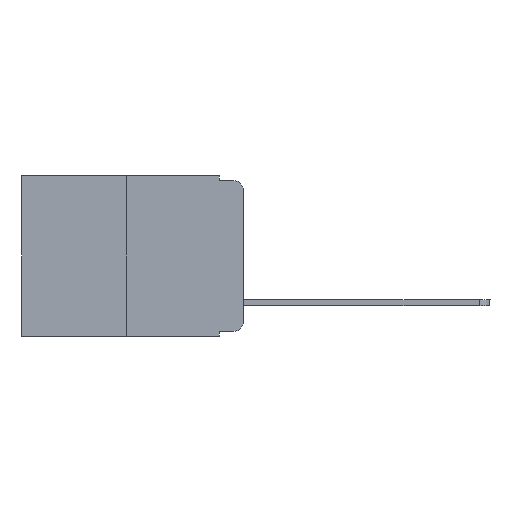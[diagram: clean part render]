
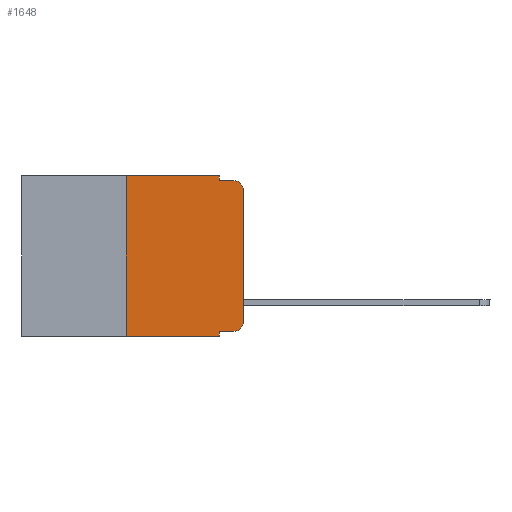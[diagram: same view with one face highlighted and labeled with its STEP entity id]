
A CAD part, left-side view. The second image highlights one B-rep face of the part: STEP entity #1648.
In plain terms, the highlighted planar face has unit normal (-1, 0, 0).
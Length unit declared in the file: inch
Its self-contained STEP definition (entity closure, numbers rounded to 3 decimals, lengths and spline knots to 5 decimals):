
#95 = LINE ( 'NONE', #11954, #1100 ) ;
#121 = VERTEX_POINT ( 'NONE', #2154 ) ;
#850 = ORIENTED_EDGE ( 'NONE', *, *, #11489, .T. ) ;
#967 = LINE ( 'NONE', #10029, #12009 ) ;
#1044 = CARTESIAN_POINT ( 'NONE',  ( 0., 0.02, -0.313 ) ) ;
#1087 = EDGE_CURVE ( 'NONE', #8851, #10928, #6207, .T. ) ;
#1100 = VECTOR ( 'NONE', #3570, 39.37008 ) ;
#1183 = VERTEX_POINT ( 'NONE', #7069 ) ;
#1648 = ADVANCED_FACE ( 'NONE', ( #4651 ), #10179, .F. ) ;
#1920 = DIRECTION ( 'NONE',  ( 0., 0., -1. ) ) ;
#1926 = AXIS2_PLACEMENT_3D ( 'NONE', #1044, #13629, #8366 ) ;
#1992 = EDGE_CURVE ( 'NONE', #7765, #7007, #9075, .T. ) ;
#2034 = EDGE_CURVE ( 'NONE', #4441, #1183, #13520, .T. ) ;
#2062 = CARTESIAN_POINT ( 'NONE',  ( 0., 0.02, -0.03 ) ) ;
#2102 = LINE ( 'NONE', #10497, #10202 ) ;
#2111 = CARTESIAN_POINT ( 'NONE',  ( 0., 0.25, 0. ) ) ;
#2154 = CARTESIAN_POINT ( 'NONE',  ( 0., 0.051, -0.333 ) ) ;
#3027 = CARTESIAN_POINT ( 'NONE',  ( 0., 0., -0.313 ) ) ;
#3145 = CARTESIAN_POINT ( 'NONE',  ( 0., 0.02, -0.333 ) ) ;
#3453 = CARTESIAN_POINT ( 'NONE',  ( 0., 0., -0.03 ) ) ;
#3570 = DIRECTION ( 'NONE',  ( 0., -1., 0. ) ) ;
#3577 = VECTOR ( 'NONE', #4311, 39.37008 ) ;
#3691 = EDGE_CURVE ( 'NONE', #121, #7007, #967, .T. ) ;
#3725 = CARTESIAN_POINT ( 'NONE',  ( 0., 0.25, -0.343 ) ) ;
#3776 = ORIENTED_EDGE ( 'NONE', *, *, #1087, .T. ) ;
#4140 = CARTESIAN_POINT ( 'NONE',  ( 0., 0.051, 0. ) ) ;
#4193 = ORIENTED_EDGE ( 'NONE', *, *, #8775, .T. ) ;
#4295 = VERTEX_POINT ( 'NONE', #4140 ) ;
#4311 = DIRECTION ( 'NONE',  ( 0., -1., 0. ) ) ;
#4322 = CARTESIAN_POINT ( 'NONE',  ( 0., 0.051, -0.01 ) ) ;
#4402 = DIRECTION ( 'NONE',  ( 0., -1., 0. ) ) ;
#4441 = VERTEX_POINT ( 'NONE', #4322 ) ;
#4563 = EDGE_CURVE ( 'NONE', #10100, #4295, #95, .T. ) ;
#4588 = ORIENTED_EDGE ( 'NONE', *, *, #13112, .T. ) ;
#4651 = FACE_OUTER_BOUND ( 'NONE', #6833, .T. ) ;
#4959 = DIRECTION ( 'NONE',  ( 0., 0., 1. ) ) ;
#5990 = CARTESIAN_POINT ( 'NONE',  ( 0., 0.051, 0. ) ) ;
#6037 = ORIENTED_EDGE ( 'NONE', *, *, #4563, .F. ) ;
#6207 = LINE ( 'NONE', #7023, #11497 ) ;
#6371 = AXIS2_PLACEMENT_3D ( 'NONE', #2062, #12422, #1920 ) ;
#6585 = ORIENTED_EDGE ( 'NONE', *, *, #3691, .F. ) ;
#6833 = EDGE_LOOP ( 'NONE', ( #3776, #4193, #12288, #9859, #6037, #12783, #11255, #6585, #850, #4588 ) ) ;
#7007 = VERTEX_POINT ( 'NONE', #10623 ) ;
#7023 = CARTESIAN_POINT ( 'NONE',  ( 0., 0., 0. ) ) ;
#7043 = DIRECTION ( 'NONE',  ( 0., 0., -1. ) ) ;
#7069 = CARTESIAN_POINT ( 'NONE',  ( 0., 0.02, -0.01 ) ) ;
#7752 = DIRECTION ( 'NONE',  ( 0., 0., -1. ) ) ;
#7765 = VERTEX_POINT ( 'NONE', #3725 ) ;
#8045 = VECTOR ( 'NONE', #7043, 39.37008 ) ;
#8288 = DIRECTION ( 'NONE',  ( 0., 0., 1. ) ) ;
#8366 = DIRECTION ( 'NONE',  ( 0., 0., -1. ) ) ;
#8600 = EDGE_CURVE ( 'NONE', #4295, #4441, #10879, .T. ) ;
#8775 = EDGE_CURVE ( 'NONE', #10928, #1183, #10866, .T. ) ;
#8794 = CARTESIAN_POINT ( 'NONE',  ( 0., 0.473, -0.343 ) ) ;
#8851 = VERTEX_POINT ( 'NONE', #3027 ) ;
#8953 = EDGE_CURVE ( 'NONE', #7765, #10100, #2102, .T. ) ;
#9075 = LINE ( 'NONE', #8794, #9766 ) ;
#9766 = VECTOR ( 'NONE', #12903, 39.37008 ) ;
#9859 = ORIENTED_EDGE ( 'NONE', *, *, #8600, .F. ) ;
#10029 = CARTESIAN_POINT ( 'NONE',  ( 0., 0.051, 0. ) ) ;
#10100 = VERTEX_POINT ( 'NONE', #2111 ) ;
#10179 = PLANE ( 'NONE',  #11096 ) ;
#10202 = VECTOR ( 'NONE', #8288, 39.37008 ) ;
#10224 = CARTESIAN_POINT ( 'NONE',  ( 0., 0.473, 0. ) ) ;
#10497 = CARTESIAN_POINT ( 'NONE',  ( 0., 0.25, 0. ) ) ;
#10623 = CARTESIAN_POINT ( 'NONE',  ( 0., 0.051, -0.343 ) ) ;
#10624 = CARTESIAN_POINT ( 'NONE',  ( 0., 0.051, -0.333 ) ) ;
#10721 = CARTESIAN_POINT ( 'NONE',  ( 0., 0.051, -0.01 ) ) ;
#10866 = CIRCLE ( 'NONE', #6371, 0.02 ) ;
#10879 = LINE ( 'NONE', #5990, #8045 ) ;
#10928 = VERTEX_POINT ( 'NONE', #3453 ) ;
#11096 = AXIS2_PLACEMENT_3D ( 'NONE', #10224, #11184, #11229 ) ;
#11184 = DIRECTION ( 'NONE',  ( 1., 0., 0. ) ) ;
#11229 = DIRECTION ( 'NONE',  ( 0., 0., -1. ) ) ;
#11255 = ORIENTED_EDGE ( 'NONE', *, *, #1992, .T. ) ;
#11489 = EDGE_CURVE ( 'NONE', #121, #12152, #11827, .T. ) ;
#11497 = VECTOR ( 'NONE', #4959, 39.37008 ) ;
#11827 = LINE ( 'NONE', #10624, #3577 ) ;
#11954 = CARTESIAN_POINT ( 'NONE',  ( 0., 0.473, 0. ) ) ;
#12009 = VECTOR ( 'NONE', #7752, 39.37008 ) ;
#12152 = VERTEX_POINT ( 'NONE', #3145 ) ;
#12253 = CIRCLE ( 'NONE', #1926, 0.02 ) ;
#12288 = ORIENTED_EDGE ( 'NONE', *, *, #2034, .F. ) ;
#12422 = DIRECTION ( 'NONE',  ( -1., 0., 0. ) ) ;
#12783 = ORIENTED_EDGE ( 'NONE', *, *, #8953, .F. ) ;
#12903 = DIRECTION ( 'NONE',  ( 0., -1., 0. ) ) ;
#13112 = EDGE_CURVE ( 'NONE', #12152, #8851, #12253, .T. ) ;
#13205 = VECTOR ( 'NONE', #4402, 39.37008 ) ;
#13520 = LINE ( 'NONE', #10721, #13205 ) ;
#13629 = DIRECTION ( 'NONE',  ( -1., 0., 0. ) ) ;
